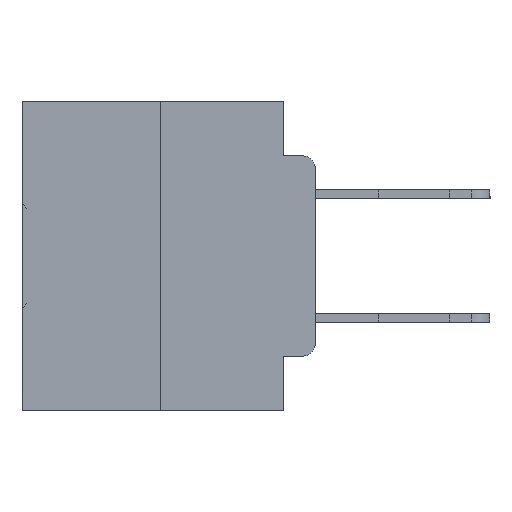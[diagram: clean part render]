
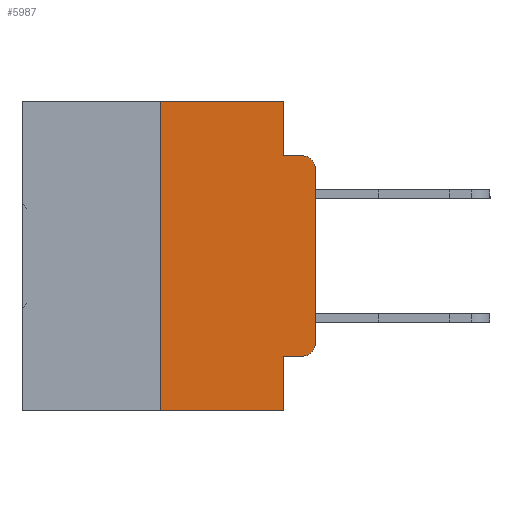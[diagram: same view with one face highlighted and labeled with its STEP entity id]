
A CAD part, left-side view. The second image highlights one B-rep face of the part: STEP entity #5987.
In plain terms, the highlighted planar face has unit normal (-1, 0, 0).
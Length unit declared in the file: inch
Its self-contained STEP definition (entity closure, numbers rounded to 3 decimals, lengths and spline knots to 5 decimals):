
#374 = DIRECTION ( 'NONE',  ( 0., -1., 0. ) ) ;
#623 = ORIENTED_EDGE ( 'NONE', *, *, #18948, .F. ) ;
#739 = LINE ( 'NONE', #3007, #28791 ) ;
#776 = CIRCLE ( 'NONE', #13277, 0.02 ) ;
#1898 = ORIENTED_EDGE ( 'NONE', *, *, #9190, .T. ) ;
#1921 = CARTESIAN_POINT ( 'NONE',  ( 0., 0.25, 0. ) ) ;
#1990 = LINE ( 'NONE', #32813, #15743 ) ;
#2278 = VERTEX_POINT ( 'NONE', #31205 ) ;
#2470 = VECTOR ( 'NONE', #20677, 39.37008 ) ;
#2801 = ORIENTED_EDGE ( 'NONE', *, *, #26786, .F. ) ;
#3007 = CARTESIAN_POINT ( 'NONE',  ( 0., 0.25, 0. ) ) ;
#3116 = DIRECTION ( 'NONE',  ( 0., 0., 1. ) ) ;
#3129 = CARTESIAN_POINT ( 'NONE',  ( 0., 0.25, -0.5 ) ) ;
#3175 = DIRECTION ( 'NONE',  ( 1., 0., 0. ) ) ;
#3270 = CARTESIAN_POINT ( 'NONE',  ( 0., 0.051, -0.4115 ) ) ;
#3320 = LINE ( 'NONE', #17957, #2470 ) ;
#4971 = ORIENTED_EDGE ( 'NONE', *, *, #33873, .F. ) ;
#5422 = EDGE_LOOP ( 'NONE', ( #1898, #28252, #623, #28690, #6741, #4971, #19941, #2801, #14455, #17854 ) ) ;
#5872 = LINE ( 'NONE', #3270, #26613 ) ;
#5987 = ADVANCED_FACE ( 'NONE', ( #28093 ), #18354, .F. ) ;
#6040 = VERTEX_POINT ( 'NONE', #3129 ) ;
#6110 = DIRECTION ( 'NONE',  ( 0., -1., 0. ) ) ;
#6598 = CARTESIAN_POINT ( 'NONE',  ( 0., 0.473, -0.5 ) ) ;
#6733 = VERTEX_POINT ( 'NONE', #12934 ) ;
#6741 = ORIENTED_EDGE ( 'NONE', *, *, #25256, .F. ) ;
#6797 = VECTOR ( 'NONE', #25489, 39.37008 ) ;
#7343 = EDGE_CURVE ( 'NONE', #2278, #16598, #776, .T. ) ;
#8507 = DIRECTION ( 'NONE',  ( -1., 0., 0. ) ) ;
#9190 = EDGE_CURVE ( 'NONE', #6733, #2278, #28343, .T. ) ;
#9885 = EDGE_CURVE ( 'NONE', #15950, #9904, #3320, .T. ) ;
#9904 = VERTEX_POINT ( 'NONE', #23368 ) ;
#9908 = LINE ( 'NONE', #6598, #30488 ) ;
#10043 = DIRECTION ( 'NONE',  ( -1., 0., 0. ) ) ;
#10544 = EDGE_CURVE ( 'NONE', #18703, #6733, #11073, .T. ) ;
#11028 = DIRECTION ( 'NONE',  ( 0., 0., -1. ) ) ;
#11073 = CIRCLE ( 'NONE', #33964, 0.02 ) ;
#12851 = VERTEX_POINT ( 'NONE', #1921 ) ;
#12934 = CARTESIAN_POINT ( 'NONE',  ( 0., 0., -0.3915 ) ) ;
#13277 = AXIS2_PLACEMENT_3D ( 'NONE', #26162, #10043, #28848 ) ;
#14175 = AXIS2_PLACEMENT_3D ( 'NONE', #18657, #3175, #11028 ) ;
#14455 = ORIENTED_EDGE ( 'NONE', *, *, #19629, .T. ) ;
#15087 = CARTESIAN_POINT ( 'NONE',  ( 0., 0.051, 0. ) ) ;
#15743 = VECTOR ( 'NONE', #374, 39.37008 ) ;
#15889 = CARTESIAN_POINT ( 'NONE',  ( 0., 0.051, -0.4115 ) ) ;
#15950 = VERTEX_POINT ( 'NONE', #15087 ) ;
#16542 = LINE ( 'NONE', #33855, #29942 ) ;
#16598 = VERTEX_POINT ( 'NONE', #28289 ) ;
#17854 = ORIENTED_EDGE ( 'NONE', *, *, #10544, .T. ) ;
#17913 = EDGE_CURVE ( 'NONE', #6040, #24115, #9908, .T. ) ;
#17957 = CARTESIAN_POINT ( 'NONE',  ( 0., 0.051, 0. ) ) ;
#18084 = VERTEX_POINT ( 'NONE', #15889 ) ;
#18354 = PLANE ( 'NONE',  #14175 ) ;
#18657 = CARTESIAN_POINT ( 'NONE',  ( 0., 0.473, 0. ) ) ;
#18703 = VERTEX_POINT ( 'NONE', #29426 ) ;
#18948 = EDGE_CURVE ( 'NONE', #9904, #16598, #26236, .T. ) ;
#19113 = DIRECTION ( 'NONE',  ( 0., -1., 0. ) ) ;
#19129 = VECTOR ( 'NONE', #19113, 39.37008 ) ;
#19629 = EDGE_CURVE ( 'NONE', #18084, #18703, #5872, .T. ) ;
#19941 = ORIENTED_EDGE ( 'NONE', *, *, #17913, .T. ) ;
#20109 = CARTESIAN_POINT ( 'NONE',  ( 0., 0., 0. ) ) ;
#20677 = DIRECTION ( 'NONE',  ( 0., 0., -1. ) ) ;
#23368 = CARTESIAN_POINT ( 'NONE',  ( 0., 0.051, -0.0885 ) ) ;
#24115 = VERTEX_POINT ( 'NONE', #28494 ) ;
#24705 = CARTESIAN_POINT ( 'NONE',  ( 0., 0.02, -0.3915 ) ) ;
#25256 = EDGE_CURVE ( 'NONE', #12851, #15950, #1990, .T. ) ;
#25489 = DIRECTION ( 'NONE',  ( 0., 0., 1. ) ) ;
#26162 = CARTESIAN_POINT ( 'NONE',  ( 0., 0.02, -0.1085 ) ) ;
#26236 = LINE ( 'NONE', #32980, #19129 ) ;
#26613 = VECTOR ( 'NONE', #6110, 39.37008 ) ;
#26786 = EDGE_CURVE ( 'NONE', #18084, #24115, #16542, .T. ) ;
#27379 = DIRECTION ( 'NONE',  ( 0., 0., -1. ) ) ;
#28093 = FACE_OUTER_BOUND ( 'NONE', #5422, .T. ) ;
#28252 = ORIENTED_EDGE ( 'NONE', *, *, #7343, .T. ) ;
#28289 = CARTESIAN_POINT ( 'NONE',  ( 0., 0.02, -0.0885 ) ) ;
#28343 = LINE ( 'NONE', #20109, #6797 ) ;
#28494 = CARTESIAN_POINT ( 'NONE',  ( 0., 0.051, -0.5 ) ) ;
#28684 = DIRECTION ( 'NONE',  ( 0., 0., -1. ) ) ;
#28690 = ORIENTED_EDGE ( 'NONE', *, *, #9885, .F. ) ;
#28791 = VECTOR ( 'NONE', #3116, 39.37008 ) ;
#28848 = DIRECTION ( 'NONE',  ( 0., 0., -1. ) ) ;
#29426 = CARTESIAN_POINT ( 'NONE',  ( 0., 0.02, -0.4115 ) ) ;
#29942 = VECTOR ( 'NONE', #28684, 39.37008 ) ;
#30488 = VECTOR ( 'NONE', #30878, 39.37008 ) ;
#30878 = DIRECTION ( 'NONE',  ( 0., -1., 0. ) ) ;
#31205 = CARTESIAN_POINT ( 'NONE',  ( 0., 0., -0.1085 ) ) ;
#32813 = CARTESIAN_POINT ( 'NONE',  ( 0., 0.473, 0. ) ) ;
#32980 = CARTESIAN_POINT ( 'NONE',  ( 0., 0.051, -0.0885 ) ) ;
#33855 = CARTESIAN_POINT ( 'NONE',  ( 0., 0.051, 0. ) ) ;
#33873 = EDGE_CURVE ( 'NONE', #6040, #12851, #739, .T. ) ;
#33964 = AXIS2_PLACEMENT_3D ( 'NONE', #24705, #8507, #27379 ) ;
